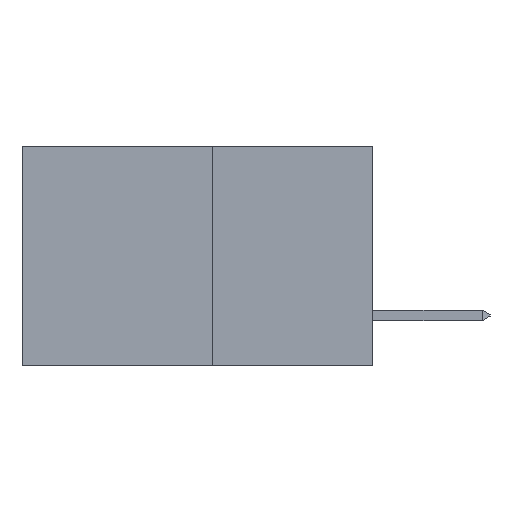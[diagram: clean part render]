
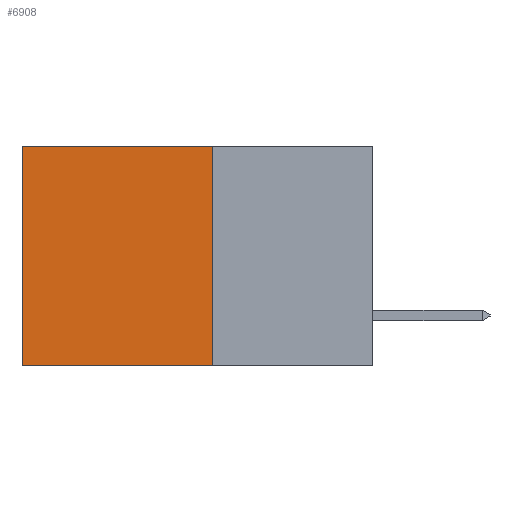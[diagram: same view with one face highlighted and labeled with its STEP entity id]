
A CAD part, left-side view. The second image highlights one B-rep face of the part: STEP entity #6908.
In plain terms, the highlighted planar face has unit normal (-1, 0, 0).
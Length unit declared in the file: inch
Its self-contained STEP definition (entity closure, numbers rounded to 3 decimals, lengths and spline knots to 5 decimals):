
#543 = LINE ( 'NONE', #13382, #13430 ) ;
#571 = ORIENTED_EDGE ( 'NONE', *, *, #9244, .T. ) ;
#821 = FACE_OUTER_BOUND ( 'NONE', #11782, .T. ) ;
#880 = LINE ( 'NONE', #12723, #4321 ) ;
#1407 = EDGE_CURVE ( 'NONE', #1559, #5208, #14039, .T. ) ;
#1559 = VERTEX_POINT ( 'NONE', #12233 ) ;
#3014 = VECTOR ( 'NONE', #4396, 39.37008 ) ;
#3226 = VERTEX_POINT ( 'NONE', #10457 ) ;
#4045 = DIRECTION ( 'NONE',  ( 0., 0., -1. ) ) ;
#4321 = VECTOR ( 'NONE', #4045, 39.37008 ) ;
#4352 = ORIENTED_EDGE ( 'NONE', *, *, #1407, .T. ) ;
#4396 = DIRECTION ( 'NONE',  ( 0., 1., 0. ) ) ;
#4498 = CARTESIAN_POINT ( 'NONE',  ( 0.277, 0.27, -0.37 ) ) ;
#4775 = CARTESIAN_POINT ( 'NONE',  ( 0.277, 0.59, -0.37 ) ) ;
#5189 = AXIS2_PLACEMENT_3D ( 'NONE', #5923, #5232, #5218 ) ;
#5208 = VERTEX_POINT ( 'NONE', #4775 ) ;
#5218 = DIRECTION ( 'NONE',  ( 0., 0., -1. ) ) ;
#5232 = DIRECTION ( 'NONE',  ( 1., 0., 0. ) ) ;
#5283 = PLANE ( 'NONE',  #5189 ) ;
#5923 = CARTESIAN_POINT ( 'NONE',  ( 0.277, 0.27, -0.37 ) ) ;
#5980 = LINE ( 'NONE', #4498, #3014 ) ;
#6908 = ADVANCED_FACE ( 'NONE', ( #821 ), #5283, .F. ) ;
#7632 = ORIENTED_EDGE ( 'NONE', *, *, #14197, .F. ) ;
#8322 = CARTESIAN_POINT ( 'NONE',  ( 0.277, 0.59, -0.37 ) ) ;
#8706 = EDGE_CURVE ( 'NONE', #11913, #5208, #5980, .T. ) ;
#8863 = DIRECTION ( 'NONE',  ( 0., 0., -1. ) ) ;
#9244 = EDGE_CURVE ( 'NONE', #3226, #1559, #543, .T. ) ;
#9332 = CARTESIAN_POINT ( 'NONE',  ( 0.277, 0.27, -0.37 ) ) ;
#9422 = ORIENTED_EDGE ( 'NONE', *, *, #8706, .F. ) ;
#10457 = CARTESIAN_POINT ( 'NONE',  ( 0.277, 0.27, 0. ) ) ;
#10863 = VECTOR ( 'NONE', #8863, 39.37008 ) ;
#11782 = EDGE_LOOP ( 'NONE', ( #4352, #9422, #7632, #571 ) ) ;
#11913 = VERTEX_POINT ( 'NONE', #9332 ) ;
#12233 = CARTESIAN_POINT ( 'NONE',  ( 0.277, 0.59, 0. ) ) ;
#12723 = CARTESIAN_POINT ( 'NONE',  ( 0.277, 0.27, -0.37 ) ) ;
#12842 = DIRECTION ( 'NONE',  ( 0., 1., 0. ) ) ;
#13382 = CARTESIAN_POINT ( 'NONE',  ( 0.277, 0.27, 0. ) ) ;
#13430 = VECTOR ( 'NONE', #12842, 39.37008 ) ;
#14039 = LINE ( 'NONE', #8322, #10863 ) ;
#14197 = EDGE_CURVE ( 'NONE', #3226, #11913, #880, .T. ) ;
